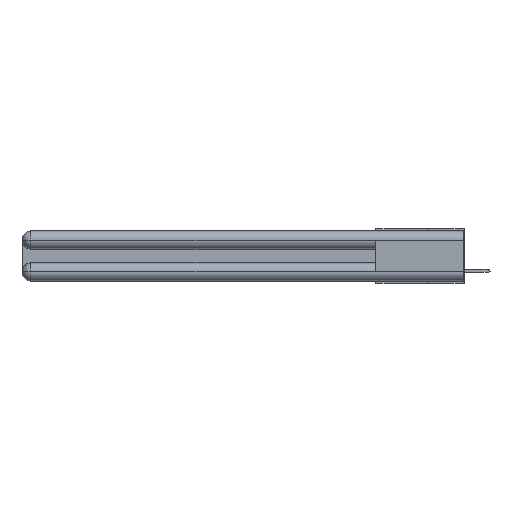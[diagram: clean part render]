
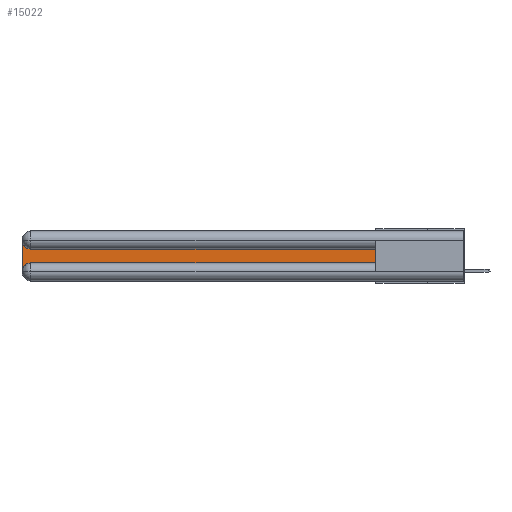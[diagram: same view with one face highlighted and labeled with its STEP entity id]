
A CAD part, left-side view. The second image highlights one B-rep face of the part: STEP entity #15022.
In plain terms, the highlighted planar face has unit normal (-1, 0, 0).
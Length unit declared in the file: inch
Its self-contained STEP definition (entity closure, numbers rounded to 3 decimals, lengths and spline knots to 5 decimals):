
#422 = ORIENTED_EDGE ( 'NONE', *, *, #9567, .T. ) ;
#1159 = VERTEX_POINT ( 'NONE', #25526 ) ;
#1466 = VECTOR ( 'NONE', #21991, 39.37008 ) ;
#2295 = CARTESIAN_POINT ( 'NONE',  ( 0.075, 3., -0.2175 ) ) ;
#2382 = EDGE_CURVE ( 'NONE', #1159, #14415, #18821, .T. ) ;
#2790 = FACE_OUTER_BOUND ( 'NONE', #4783, .T. ) ;
#2993 = DIRECTION ( 'NONE',  ( 0., -1., 0. ) ) ;
#3736 = CARTESIAN_POINT ( 'NONE',  ( 0.075, 2.94, -0.1225 ) ) ;
#4327 = DIRECTION ( 'NONE',  ( 1., 0., 0. ) ) ;
#4420 = DIRECTION ( 'NONE',  ( 0., 0., -1. ) ) ;
#4600 = ORIENTED_EDGE ( 'NONE', *, *, #23219, .T. ) ;
#4783 = EDGE_LOOP ( 'NONE', ( #25575, #22704, #15723, #422, #4600, #16138 ) ) ;
#5350 = CIRCLE ( 'NONE', #11286, 0.06 ) ;
#6789 = LINE ( 'NONE', #14166, #1466 ) ;
#9567 = EDGE_CURVE ( 'NONE', #14415, #10079, #5350, .T. ) ;
#10079 = VERTEX_POINT ( 'NONE', #11745 ) ;
#10458 = PLANE ( 'NONE',  #23398 ) ;
#11286 = AXIS2_PLACEMENT_3D ( 'NONE', #20077, #4327, #4420 ) ;
#11745 = CARTESIAN_POINT ( 'NONE',  ( 0.075, 2.94, -0.2175 ) ) ;
#11779 = CARTESIAN_POINT ( 'NONE',  ( 0.075, 0.6, -0.2175 ) ) ;
#12015 = EDGE_CURVE ( 'NONE', #13990, #1159, #16193, .T. ) ;
#12448 = DIRECTION ( 'NONE',  ( 0., 0., -1. ) ) ;
#13605 = EDGE_CURVE ( 'NONE', #13861, #13990, #20149, .T. ) ;
#13759 = CARTESIAN_POINT ( 'NONE',  ( 0.075, 0.6, -0.1225 ) ) ;
#13803 = VECTOR ( 'NONE', #12448, 39.37008 ) ;
#13861 = VERTEX_POINT ( 'NONE', #13759 ) ;
#13894 = CARTESIAN_POINT ( 'NONE',  ( 0.075, 0.6, -0.2175 ) ) ;
#13990 = VERTEX_POINT ( 'NONE', #3736 ) ;
#14166 = CARTESIAN_POINT ( 'NONE',  ( 0.075, 0.6, -0.2175 ) ) ;
#14186 = CARTESIAN_POINT ( 'NONE',  ( 0.075, 3., -0.1225 ) ) ;
#14415 = VERTEX_POINT ( 'NONE', #16747 ) ;
#14497 = CARTESIAN_POINT ( 'NONE',  ( 0.075, 0.6, -0.1225 ) ) ;
#14862 = VECTOR ( 'NONE', #18163, 39.37008 ) ;
#15022 = ADVANCED_FACE ( 'NONE', ( #2790 ), #10458, .F. ) ;
#15390 = AXIS2_PLACEMENT_3D ( 'NONE', #23147, #21156, #21237 ) ;
#15723 = ORIENTED_EDGE ( 'NONE', *, *, #2382, .T. ) ;
#16138 = ORIENTED_EDGE ( 'NONE', *, *, #21807, .T. ) ;
#16193 = CIRCLE ( 'NONE', #15390, 0.06 ) ;
#16369 = VERTEX_POINT ( 'NONE', #11779 ) ;
#16557 = DIRECTION ( 'NONE',  ( 1., 0., 0. ) ) ;
#16747 = CARTESIAN_POINT ( 'NONE',  ( 0.075, 3., -0.2775 ) ) ;
#18163 = DIRECTION ( 'NONE',  ( 0., 1., 0. ) ) ;
#18821 = LINE ( 'NONE', #2295, #13803 ) ;
#20077 = CARTESIAN_POINT ( 'NONE',  ( 0.075, 2.94, -0.2775 ) ) ;
#20149 = LINE ( 'NONE', #14497, #14862 ) ;
#21051 = VECTOR ( 'NONE', #2993, 39.37008 ) ;
#21156 = DIRECTION ( 'NONE',  ( 1., 0., 0. ) ) ;
#21237 = DIRECTION ( 'NONE',  ( 0., 0., -1. ) ) ;
#21807 = EDGE_CURVE ( 'NONE', #16369, #13861, #6789, .T. ) ;
#21991 = DIRECTION ( 'NONE',  ( 0., 0., 1. ) ) ;
#22704 = ORIENTED_EDGE ( 'NONE', *, *, #12015, .T. ) ;
#23147 = CARTESIAN_POINT ( 'NONE',  ( 0.075, 2.94, -0.0625 ) ) ;
#23219 = EDGE_CURVE ( 'NONE', #10079, #16369, #25748, .T. ) ;
#23398 = AXIS2_PLACEMENT_3D ( 'NONE', #14186, #16557, #24274 ) ;
#24274 = DIRECTION ( 'NONE',  ( 0., 0., -1. ) ) ;
#25526 = CARTESIAN_POINT ( 'NONE',  ( 0.075, 3., -0.0625 ) ) ;
#25575 = ORIENTED_EDGE ( 'NONE', *, *, #13605, .T. ) ;
#25748 = LINE ( 'NONE', #13894, #21051 ) ;
